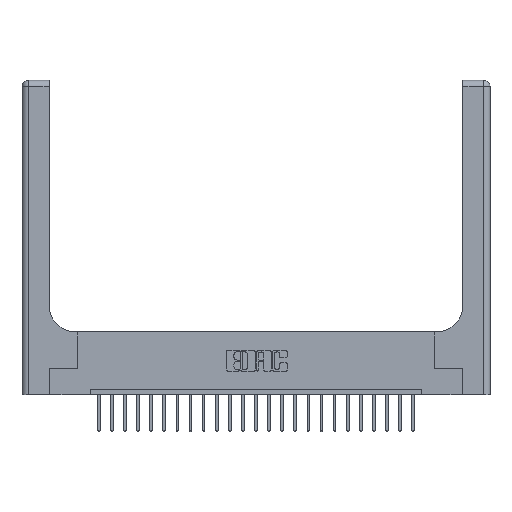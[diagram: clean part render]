
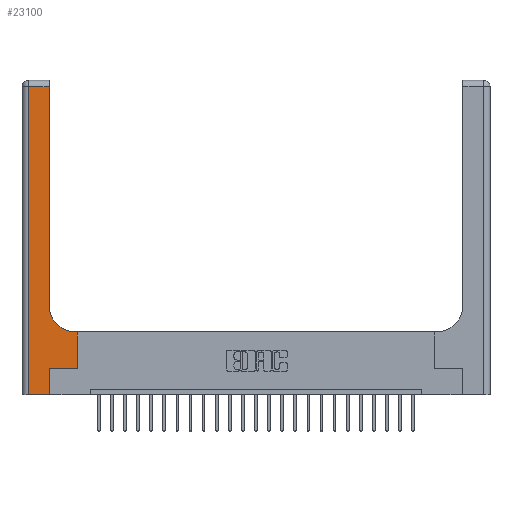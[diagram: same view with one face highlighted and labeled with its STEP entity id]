
A CAD part, top view. The second image highlights one B-rep face of the part: STEP entity #23100.
In plain terms, the highlighted planar face has unit normal (0, 0, 1).
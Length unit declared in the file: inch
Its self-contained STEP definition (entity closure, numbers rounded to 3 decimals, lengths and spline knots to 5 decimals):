
#560 = DIRECTION ( 'NONE',  ( 0., -1., 0. ) ) ;
#792 = EDGE_CURVE ( 'NONE', #21410, #3736, #21243, .T. ) ;
#1015 = DIRECTION ( 'NONE',  ( 0., 0., -1. ) ) ;
#1429 = DIRECTION ( 'NONE',  ( 1., 0., 0. ) ) ;
#1666 = ORIENTED_EDGE ( 'NONE', *, *, #18200, .T. ) ;
#1939 = DIRECTION ( 'NONE',  ( 1., 0., 0. ) ) ;
#2244 = DIRECTION ( 'NONE',  ( 0., 1., 0. ) ) ;
#2895 = CARTESIAN_POINT ( 'NONE',  ( 0.06, 0., 0.37 ) ) ;
#3217 = EDGE_CURVE ( 'NONE', #3736, #7740, #7879, .T. ) ;
#3607 = CARTESIAN_POINT ( 'NONE',  ( 0.265, 0.25, 0.37 ) ) ;
#3702 = DIRECTION ( 'NONE',  ( -1., 0., 0. ) ) ;
#3736 = VERTEX_POINT ( 'NONE', #14713 ) ;
#4170 = VECTOR ( 'NONE', #1939, 39.37008 ) ;
#4750 = CARTESIAN_POINT ( 'NONE',  ( 0.528, 0.6, 0.37 ) ) ;
#4755 = CARTESIAN_POINT ( 'NONE',  ( 0., 0., 0.37 ) ) ;
#5015 = VECTOR ( 'NONE', #1429, 39.37008 ) ;
#5128 = VERTEX_POINT ( 'NONE', #6310 ) ;
#5860 = DIRECTION ( 'NONE',  ( 0., 1., 0. ) ) ;
#6310 = CARTESIAN_POINT ( 'NONE',  ( 0.528, 0.25, 0.37 ) ) ;
#6323 = EDGE_LOOP ( 'NONE', ( #6911, #16473, #13582, #14598, #18890, #7722, #1666, #16875, #6742 ) ) ;
#6601 = DIRECTION ( 'NONE',  ( 1., 0., 0. ) ) ;
#6742 = ORIENTED_EDGE ( 'NONE', *, *, #10549, .T. ) ;
#6911 = ORIENTED_EDGE ( 'NONE', *, *, #20155, .T. ) ;
#6987 = LINE ( 'NONE', #17526, #10722 ) ;
#7211 = VECTOR ( 'NONE', #2244, 39.37008 ) ;
#7722 = ORIENTED_EDGE ( 'NONE', *, *, #8790, .T. ) ;
#7740 = VERTEX_POINT ( 'NONE', #10114 ) ;
#7831 = CARTESIAN_POINT ( 'NONE',  ( 0.51, 0.6, 0.37 ) ) ;
#7879 = LINE ( 'NONE', #22336, #22114 ) ;
#8597 = CARTESIAN_POINT ( 'NONE',  ( 0., 3., 0.37 ) ) ;
#8790 = EDGE_CURVE ( 'NONE', #7740, #5128, #16277, .T. ) ;
#8793 = VECTOR ( 'NONE', #12769, 39.37008 ) ;
#8796 = CARTESIAN_POINT ( 'NONE',  ( 0.06, 2.94, 0.37 ) ) ;
#9257 = CARTESIAN_POINT ( 'NONE',  ( 0.26, 0.85, 0.37 ) ) ;
#10114 = CARTESIAN_POINT ( 'NONE',  ( 0.265, 0.25, 0.37 ) ) ;
#10251 = LINE ( 'NONE', #13250, #14866 ) ;
#10481 = FACE_OUTER_BOUND ( 'NONE', #6323, .T. ) ;
#10549 = EDGE_CURVE ( 'NONE', #13113, #18072, #21481, .T. ) ;
#10722 = VECTOR ( 'NONE', #19315, 39.37008 ) ;
#10886 = VERTEX_POINT ( 'NONE', #4750 ) ;
#11145 = AXIS2_PLACEMENT_3D ( 'NONE', #8597, #12158, #15580 ) ;
#11383 = CARTESIAN_POINT ( 'NONE',  ( 0.528, 0.25, 0.37 ) ) ;
#12158 = DIRECTION ( 'NONE',  ( 0., 0., -1. ) ) ;
#12769 = DIRECTION ( 'NONE',  ( 0., 1., 0. ) ) ;
#12823 = LINE ( 'NONE', #16364, #13674 ) ;
#13113 = VERTEX_POINT ( 'NONE', #7831 ) ;
#13250 = CARTESIAN_POINT ( 'NONE',  ( 0.06, 3., 0.37 ) ) ;
#13582 = ORIENTED_EDGE ( 'NONE', *, *, #21340, .T. ) ;
#13674 = VECTOR ( 'NONE', #3702, 39.37008 ) ;
#14032 = VERTEX_POINT ( 'NONE', #8796 ) ;
#14292 = LINE ( 'NONE', #14412, #8793 ) ;
#14412 = CARTESIAN_POINT ( 'NONE',  ( 0.26, 3., 0.37 ) ) ;
#14598 = ORIENTED_EDGE ( 'NONE', *, *, #792, .T. ) ;
#14713 = CARTESIAN_POINT ( 'NONE',  ( 0.265, 0., 0.37 ) ) ;
#14866 = VECTOR ( 'NONE', #560, 39.37008 ) ;
#15282 = LINE ( 'NONE', #11383, #7211 ) ;
#15580 = DIRECTION ( 'NONE',  ( -1., 0., 0. ) ) ;
#15845 = CARTESIAN_POINT ( 'NONE',  ( 0.26, 2.94, 0.37 ) ) ;
#16277 = LINE ( 'NONE', #3607, #4170 ) ;
#16364 = CARTESIAN_POINT ( 'NONE',  ( 0., 2.94, 0.37 ) ) ;
#16473 = ORIENTED_EDGE ( 'NONE', *, *, #19290, .T. ) ;
#16875 = ORIENTED_EDGE ( 'NONE', *, *, #21025, .T. ) ;
#17526 = CARTESIAN_POINT ( 'NONE',  ( 0.26, 0.6, 0.37 ) ) ;
#18072 = VERTEX_POINT ( 'NONE', #9257 ) ;
#18200 = EDGE_CURVE ( 'NONE', #5128, #10886, #15282, .T. ) ;
#18890 = ORIENTED_EDGE ( 'NONE', *, *, #3217, .T. ) ;
#19290 = EDGE_CURVE ( 'NONE', #22668, #14032, #12823, .T. ) ;
#19315 = DIRECTION ( 'NONE',  ( -1., 0., 0. ) ) ;
#20155 = EDGE_CURVE ( 'NONE', #18072, #22668, #14292, .T. ) ;
#21025 = EDGE_CURVE ( 'NONE', #10886, #13113, #6987, .T. ) ;
#21243 = LINE ( 'NONE', #4755, #5015 ) ;
#21340 = EDGE_CURVE ( 'NONE', #14032, #21410, #10251, .T. ) ;
#21410 = VERTEX_POINT ( 'NONE', #2895 ) ;
#21481 = CIRCLE ( 'NONE', #22614, 0.25 ) ;
#22114 = VECTOR ( 'NONE', #5860, 39.37008 ) ;
#22336 = CARTESIAN_POINT ( 'NONE',  ( 0.265, 0., 0.37 ) ) ;
#22614 = AXIS2_PLACEMENT_3D ( 'NONE', #22838, #1015, #6601 ) ;
#22668 = VERTEX_POINT ( 'NONE', #15845 ) ;
#22825 = PLANE ( 'NONE',  #11145 ) ;
#22838 = CARTESIAN_POINT ( 'NONE',  ( 0.51, 0.85, 0.37 ) ) ;
#23100 = ADVANCED_FACE ( 'NONE', ( #10481 ), #22825, .F. ) ;
